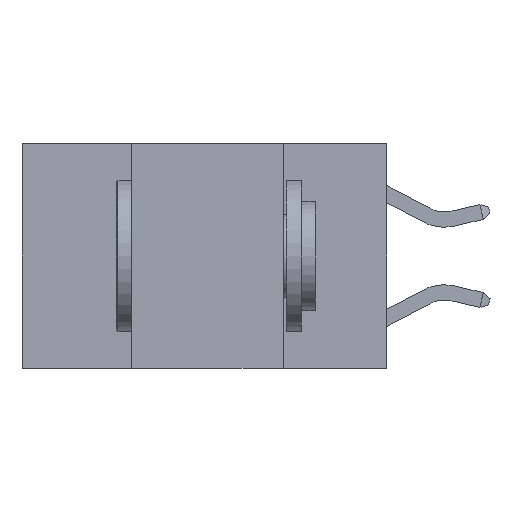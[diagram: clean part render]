
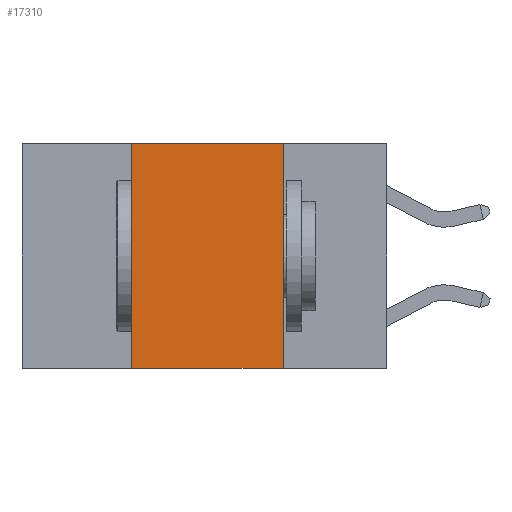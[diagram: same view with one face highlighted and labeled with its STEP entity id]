
A CAD part, left-side view. The second image highlights one B-rep face of the part: STEP entity #17310.
In plain terms, the highlighted planar face has unit normal (-1, 0, 0).
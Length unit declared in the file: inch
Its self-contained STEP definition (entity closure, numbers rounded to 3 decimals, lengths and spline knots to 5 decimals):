
#241 = EDGE_CURVE ( 'NONE', #3196, #20726, #14553, .T. ) ;
#723 = EDGE_CURVE ( 'NONE', #17595, #20726, #18599, .T. ) ;
#1872 = DIRECTION ( 'NONE',  ( 0., -1., 0. ) ) ;
#2142 = AXIS2_PLACEMENT_3D ( 'NONE', #6888, #16095, #9227 ) ;
#2176 = CARTESIAN_POINT ( 'NONE',  ( 0., 0.42, 0. ) ) ;
#2185 = EDGE_CURVE ( 'NONE', #17595, #8172, #9156, .T. ) ;
#2859 = DIRECTION ( 'NONE',  ( 0., 0., 1. ) ) ;
#3196 = VERTEX_POINT ( 'NONE', #19380 ) ;
#3934 = ORIENTED_EDGE ( 'NONE', *, *, #241, .F. ) ;
#6888 = CARTESIAN_POINT ( 'NONE',  ( 0., 0.6, 0. ) ) ;
#7003 = VECTOR ( 'NONE', #25169, 39.37008 ) ;
#8172 = VERTEX_POINT ( 'NONE', #2176 ) ;
#8226 = VECTOR ( 'NONE', #1872, 39.37008 ) ;
#8462 = LINE ( 'NONE', #28465, #8226 ) ;
#9156 = LINE ( 'NONE', #22869, #10747 ) ;
#9227 = DIRECTION ( 'NONE',  ( 0., 0., -1. ) ) ;
#10747 = VECTOR ( 'NONE', #2859, 39.37008 ) ;
#11776 = EDGE_CURVE ( 'NONE', #8172, #3196, #8462, .T. ) ;
#14278 = ORIENTED_EDGE ( 'NONE', *, *, #11776, .F. ) ;
#14553 = LINE ( 'NONE', #16874, #26853 ) ;
#14691 = FACE_OUTER_BOUND ( 'NONE', #17783, .T. ) ;
#15824 = CARTESIAN_POINT ( 'NONE',  ( 0., 0.17, -0.37 ) ) ;
#16095 = DIRECTION ( 'NONE',  ( 1., 0., 0. ) ) ;
#16874 = CARTESIAN_POINT ( 'NONE',  ( 0., 0.17, 0. ) ) ;
#17310 = ADVANCED_FACE ( 'NONE', ( #14691 ), #25134, .F. ) ;
#17595 = VERTEX_POINT ( 'NONE', #23654 ) ;
#17783 = EDGE_LOOP ( 'NONE', ( #3934, #14278, #19947, #22696 ) ) ;
#18599 = LINE ( 'NONE', #21213, #7003 ) ;
#19380 = CARTESIAN_POINT ( 'NONE',  ( 0., 0.17, 0. ) ) ;
#19947 = ORIENTED_EDGE ( 'NONE', *, *, #2185, .F. ) ;
#20726 = VERTEX_POINT ( 'NONE', #15824 ) ;
#20965 = DIRECTION ( 'NONE',  ( 0., 0., -1. ) ) ;
#21213 = CARTESIAN_POINT ( 'NONE',  ( 0., 0.6, -0.37 ) ) ;
#22696 = ORIENTED_EDGE ( 'NONE', *, *, #723, .T. ) ;
#22869 = CARTESIAN_POINT ( 'NONE',  ( 0., 0.42, 0. ) ) ;
#23654 = CARTESIAN_POINT ( 'NONE',  ( 0., 0.42, -0.37 ) ) ;
#25134 = PLANE ( 'NONE',  #2142 ) ;
#25169 = DIRECTION ( 'NONE',  ( 0., -1., 0. ) ) ;
#26853 = VECTOR ( 'NONE', #20965, 39.37008 ) ;
#28465 = CARTESIAN_POINT ( 'NONE',  ( 0., 0.6, 0. ) ) ;
